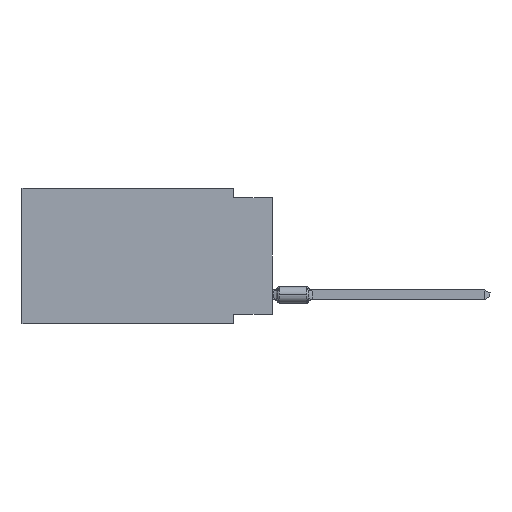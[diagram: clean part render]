
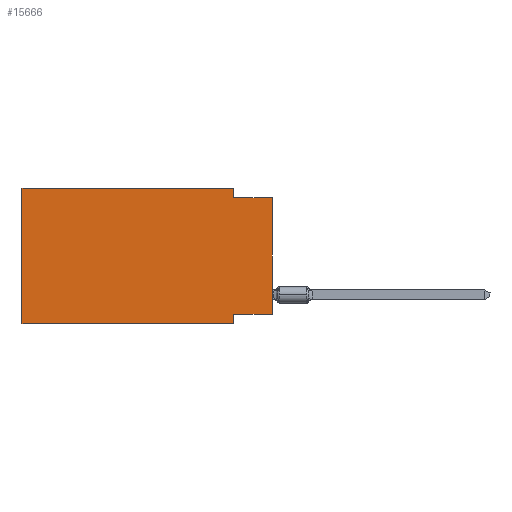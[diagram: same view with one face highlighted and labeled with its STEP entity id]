
A CAD part, left-side view. The second image highlights one B-rep face of the part: STEP entity #15666.
In plain terms, the highlighted planar face has unit normal (-1, 0, 0).
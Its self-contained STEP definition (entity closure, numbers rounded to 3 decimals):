
#960 = EDGE_CURVE ( 'NONE', #3599, #32906, #11949, .T. ) ;
#1442 = CARTESIAN_POINT ( 'NONE',  ( 0., 16.383, 0. ) ) ;
#1959 = ORIENTED_EDGE ( 'NONE', *, *, #22464, .F. ) ;
#2085 = EDGE_LOOP ( 'NONE', ( #26162, #4447, #10307, #35281, #22414, #4029, #7295, #1959 ) ) ;
#2874 = VECTOR ( 'NONE', #39608, 1000. ) ;
#3082 = CARTESIAN_POINT ( 'NONE',  ( 0., 16.383, -8.89 ) ) ;
#3357 = LINE ( 'NONE', #38920, #10066 ) ;
#3599 = VERTEX_POINT ( 'NONE', #17119 ) ;
#3752 = AXIS2_PLACEMENT_3D ( 'NONE', #14468, #8272, #18285 ) ;
#4029 = ORIENTED_EDGE ( 'NONE', *, *, #6289, .T. ) ;
#4447 = ORIENTED_EDGE ( 'NONE', *, *, #960, .F. ) ;
#4844 = EDGE_CURVE ( 'NONE', #41717, #3599, #27374, .T. ) ;
#5274 = VECTOR ( 'NONE', #16041, 1000. ) ;
#5666 = CARTESIAN_POINT ( 'NONE',  ( 0., 2.54, -8.255 ) ) ;
#6289 = EDGE_CURVE ( 'NONE', #37589, #38715, #25661, .T. ) ;
#6631 = EDGE_CURVE ( 'NONE', #20954, #32906, #22008, .T. ) ;
#7295 = ORIENTED_EDGE ( 'NONE', *, *, #41032, .F. ) ;
#8272 = DIRECTION ( 'NONE',  ( 1., 0., 0. ) ) ;
#8900 = VECTOR ( 'NONE', #31032, 1000. ) ;
#10066 = VECTOR ( 'NONE', #16155, 1000. ) ;
#10307 = ORIENTED_EDGE ( 'NONE', *, *, #4844, .F. ) ;
#11757 = VERTEX_POINT ( 'NONE', #5666 ) ;
#11949 = LINE ( 'NONE', #40892, #27327 ) ;
#14468 = CARTESIAN_POINT ( 'NONE',  ( 0., 16.383, 0. ) ) ;
#14650 = CARTESIAN_POINT ( 'NONE',  ( 0., 0., -0.635 ) ) ;
#15358 = CARTESIAN_POINT ( 'NONE',  ( 0., 2.54, 0. ) ) ;
#15666 = ADVANCED_FACE ( 'NONE', ( #37017 ), #17871, .F. ) ;
#16041 = DIRECTION ( 'NONE',  ( 0., 0., 1. ) ) ;
#16155 = DIRECTION ( 'NONE',  ( 0., 0., 1. ) ) ;
#16303 = DIRECTION ( 'NONE',  ( 0., -1., 0. ) ) ;
#17119 = CARTESIAN_POINT ( 'NONE',  ( 0., 2.54, -0.635 ) ) ;
#17782 = DIRECTION ( 'NONE',  ( 0., 0., -1. ) ) ;
#17871 = PLANE ( 'NONE',  #3752 ) ;
#18051 = CARTESIAN_POINT ( 'NONE',  ( 0., 0., -8.255 ) ) ;
#18285 = DIRECTION ( 'NONE',  ( 0., 0., -1. ) ) ;
#20954 = VERTEX_POINT ( 'NONE', #32312 ) ;
#21319 = DIRECTION ( 'NONE',  ( 0., -1., 0. ) ) ;
#22008 = LINE ( 'NONE', #34989, #5274 ) ;
#22414 = ORIENTED_EDGE ( 'NONE', *, *, #32702, .F. ) ;
#22464 = EDGE_CURVE ( 'NONE', #20954, #11757, #25476, .T. ) ;
#23759 = CARTESIAN_POINT ( 'NONE',  ( 0., 16.383, -8.89 ) ) ;
#24503 = EDGE_CURVE ( 'NONE', #28414, #41717, #29830, .T. ) ;
#25476 = LINE ( 'NONE', #18051, #8900 ) ;
#25661 = LINE ( 'NONE', #3082, #41276 ) ;
#26162 = ORIENTED_EDGE ( 'NONE', *, *, #6631, .T. ) ;
#26932 = LINE ( 'NONE', #36296, #40791 ) ;
#27327 = VECTOR ( 'NONE', #21319, 1000. ) ;
#27374 = LINE ( 'NONE', #30558, #33059 ) ;
#28414 = VERTEX_POINT ( 'NONE', #1442 ) ;
#29615 = CARTESIAN_POINT ( 'NONE',  ( 0., 16.383, 0. ) ) ;
#29830 = LINE ( 'NONE', #29615, #2874 ) ;
#30558 = CARTESIAN_POINT ( 'NONE',  ( 0., 2.54, 0. ) ) ;
#31032 = DIRECTION ( 'NONE',  ( 0., 1., 0. ) ) ;
#32312 = CARTESIAN_POINT ( 'NONE',  ( 0., 0., -8.255 ) ) ;
#32702 = EDGE_CURVE ( 'NONE', #37589, #28414, #3357, .T. ) ;
#32906 = VERTEX_POINT ( 'NONE', #14650 ) ;
#33059 = VECTOR ( 'NONE', #17782, 1000. ) ;
#33313 = DIRECTION ( 'NONE',  ( 0., 0., -1. ) ) ;
#33561 = CARTESIAN_POINT ( 'NONE',  ( 0., 2.54, -8.89 ) ) ;
#34989 = CARTESIAN_POINT ( 'NONE',  ( 0., 0., 0. ) ) ;
#35281 = ORIENTED_EDGE ( 'NONE', *, *, #24503, .F. ) ;
#36296 = CARTESIAN_POINT ( 'NONE',  ( 0., 2.54, -8.89 ) ) ;
#37017 = FACE_OUTER_BOUND ( 'NONE', #2085, .T. ) ;
#37589 = VERTEX_POINT ( 'NONE', #23759 ) ;
#38715 = VERTEX_POINT ( 'NONE', #33561 ) ;
#38920 = CARTESIAN_POINT ( 'NONE',  ( 0., 16.383, 0. ) ) ;
#39608 = DIRECTION ( 'NONE',  ( 0., -1., 0. ) ) ;
#40791 = VECTOR ( 'NONE', #33313, 1000. ) ;
#40892 = CARTESIAN_POINT ( 'NONE',  ( 0., 0., -0.635 ) ) ;
#41032 = EDGE_CURVE ( 'NONE', #11757, #38715, #26932, .T. ) ;
#41276 = VECTOR ( 'NONE', #16303, 1000. ) ;
#41717 = VERTEX_POINT ( 'NONE', #15358 ) ;
